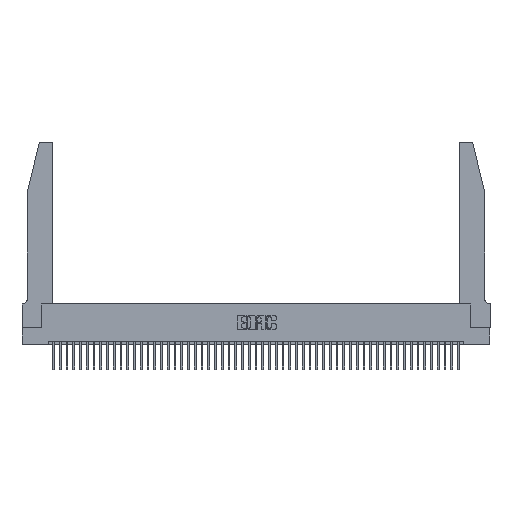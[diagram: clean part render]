
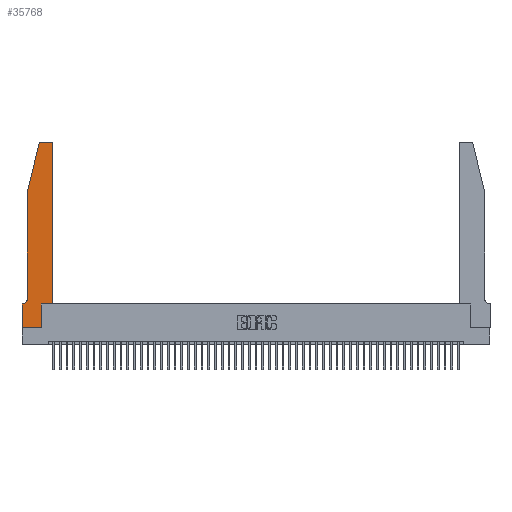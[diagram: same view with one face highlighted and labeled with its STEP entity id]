
A CAD part, top view. The second image highlights one B-rep face of the part: STEP entity #35768.
In plain terms, the highlighted planar face has unit normal (0, 0, 1).
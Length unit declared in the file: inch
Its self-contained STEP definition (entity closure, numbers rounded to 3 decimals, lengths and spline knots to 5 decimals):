
#650 = CARTESIAN_POINT ( 'NONE',  ( 0.0055, 0.42, 0.37 ) ) ;
#832 = CIRCLE ( 'NONE', #42699, 0.03 ) ;
#855 = DIRECTION ( 'NONE',  ( 1., 0., 0. ) ) ;
#888 = CARTESIAN_POINT ( 'NONE',  ( 0.284, 2.75, 0.37 ) ) ;
#952 = VERTEX_POINT ( 'NONE', #888 ) ;
#1304 = VERTEX_POINT ( 'NONE', #30046 ) ;
#1412 = VECTOR ( 'NONE', #47575, 39.37008 ) ;
#1916 = VECTOR ( 'NONE', #10757, 39.37008 ) ;
#2105 = CARTESIAN_POINT ( 'NONE',  ( 0., 0.35, 0.37 ) ) ;
#2671 = DIRECTION ( 'NONE',  ( 1., 0., 0. ) ) ;
#4132 = CARTESIAN_POINT ( 'NONE',  ( 0.0755, 2., 0.37 ) ) ;
#4643 = DIRECTION ( 'NONE',  ( -1., 0., 0. ) ) ;
#5160 = VERTEX_POINT ( 'NONE', #36260 ) ;
#5550 = ORIENTED_EDGE ( 'NONE', *, *, #30236, .T. ) ;
#7362 = CARTESIAN_POINT ( 'NONE',  ( 0.25487, 2.72718, 0.37 ) ) ;
#9404 = VERTEX_POINT ( 'NONE', #39315 ) ;
#9536 = CARTESIAN_POINT ( 'NONE',  ( 0.4205, 2.72, 0.37 ) ) ;
#9653 = AXIS2_PLACEMENT_3D ( 'NONE', #47207, #24166, #855 ) ;
#10757 = DIRECTION ( 'NONE',  ( -1., 0., 0. ) ) ;
#10974 = ORIENTED_EDGE ( 'NONE', *, *, #25733, .T. ) ;
#11867 = LINE ( 'NONE', #12893, #1412 ) ;
#12607 = FACE_OUTER_BOUND ( 'NONE', #40904, .T. ) ;
#12893 = CARTESIAN_POINT ( 'NONE',  ( 0.2865, 0.35, 0.37 ) ) ;
#13174 = LINE ( 'NONE', #13328, #23443 ) ;
#13272 = CARTESIAN_POINT ( 'NONE',  ( 0.0755, 0.42, 0.37 ) ) ;
#13328 = CARTESIAN_POINT ( 'NONE',  ( 0.4505, 0.35, 0.37 ) ) ;
#13420 = DIRECTION ( 'NONE',  ( 1., 0., 0. ) ) ;
#13622 = ORIENTED_EDGE ( 'NONE', *, *, #49044, .T. ) ;
#13881 = VERTEX_POINT ( 'NONE', #47360 ) ;
#14043 = DIRECTION ( 'NONE',  ( 0., -1., 0. ) ) ;
#14180 = AXIS2_PLACEMENT_3D ( 'NONE', #2105, #44714, #21693 ) ;
#14800 = DIRECTION ( 'NONE',  ( 0., -1., 0. ) ) ;
#15690 = LINE ( 'NONE', #17488, #34949 ) ;
#16116 = VERTEX_POINT ( 'NONE', #21688 ) ;
#16924 = VERTEX_POINT ( 'NONE', #7362 ) ;
#17362 = CIRCLE ( 'NONE', #27234, 0.07 ) ;
#17374 = EDGE_CURVE ( 'NONE', #13881, #32574, #44291, .T. ) ;
#17488 = CARTESIAN_POINT ( 'NONE',  ( 0.2605, 2.75, 0.37 ) ) ;
#17783 = VERTEX_POINT ( 'NONE', #44051 ) ;
#18094 = VERTEX_POINT ( 'NONE', #34466 ) ;
#18521 = CARTESIAN_POINT ( 'NONE',  ( 0.0755, 0.35, 0.37 ) ) ;
#18881 = CIRCLE ( 'NONE', #9653, 0.03 ) ;
#19479 = ORIENTED_EDGE ( 'NONE', *, *, #36534, .T. ) ;
#20086 = EDGE_CURVE ( 'NONE', #44939, #952, #15690, .T. ) ;
#20116 = ORIENTED_EDGE ( 'NONE', *, *, #33335, .T. ) ;
#20129 = LINE ( 'NONE', #48945, #21354 ) ;
#21072 = EDGE_CURVE ( 'NONE', #17783, #5160, #13174, .T. ) ;
#21112 = DIRECTION ( 'NONE',  ( 1., 0., 0. ) ) ;
#21149 = CARTESIAN_POINT ( 'NONE',  ( 0.4205, 2.75, 0.37 ) ) ;
#21354 = VECTOR ( 'NONE', #2671, 39.37008 ) ;
#21688 = CARTESIAN_POINT ( 'NONE',  ( 0., 0., 0.37 ) ) ;
#21693 = DIRECTION ( 'NONE',  ( 1., 0., 0. ) ) ;
#22400 = CARTESIAN_POINT ( 'NONE',  ( 0.0755, 2., 0.37 ) ) ;
#23443 = VECTOR ( 'NONE', #21112, 39.37008 ) ;
#23466 = DIRECTION ( 'NONE',  ( -0.239, -0.971, 0. ) ) ;
#24165 = VECTOR ( 'NONE', #23466, 39.37008 ) ;
#24166 = DIRECTION ( 'NONE',  ( 0., 0., 1. ) ) ;
#24174 = CARTESIAN_POINT ( 'NONE',  ( 0., 0.35, 0.37 ) ) ;
#24873 = VECTOR ( 'NONE', #25660, 39.37008 ) ;
#24995 = VERTEX_POINT ( 'NONE', #13272 ) ;
#25513 = CARTESIAN_POINT ( 'NONE',  ( 0., 0., 0.37 ) ) ;
#25660 = DIRECTION ( 'NONE',  ( 0., 1., 0. ) ) ;
#25733 = EDGE_CURVE ( 'NONE', #32574, #16116, #36470, .T. ) ;
#27234 = AXIS2_PLACEMENT_3D ( 'NONE', #650, #27822, #4643 ) ;
#27822 = DIRECTION ( 'NONE',  ( 0., 0., -1. ) ) ;
#27868 = ORIENTED_EDGE ( 'NONE', *, *, #49334, .T. ) ;
#28669 = VECTOR ( 'NONE', #14043, 39.37008 ) ;
#30046 = CARTESIAN_POINT ( 'NONE',  ( 0.2865, 0., 0.37 ) ) ;
#30100 = EDGE_CURVE ( 'NONE', #24995, #13881, #17362, .T. ) ;
#30236 = EDGE_CURVE ( 'NONE', #18094, #44939, #832, .T. ) ;
#32574 = VERTEX_POINT ( 'NONE', #24174 ) ;
#32898 = ORIENTED_EDGE ( 'NONE', *, *, #47978, .T. ) ;
#33335 = EDGE_CURVE ( 'NONE', #16116, #1304, #20129, .T. ) ;
#34466 = CARTESIAN_POINT ( 'NONE',  ( 0.4505, 2.72, 0.37 ) ) ;
#34949 = VECTOR ( 'NONE', #36811, 39.37008 ) ;
#35097 = ORIENTED_EDGE ( 'NONE', *, *, #21072, .T. ) ;
#35347 = ORIENTED_EDGE ( 'NONE', *, *, #20086, .T. ) ;
#35684 = ORIENTED_EDGE ( 'NONE', *, *, #17374, .T. ) ;
#35768 = ADVANCED_FACE ( 'NONE', ( #12607 ), #36949, .T. ) ;
#36260 = CARTESIAN_POINT ( 'NONE',  ( 0.4505, 0.35, 0.37 ) ) ;
#36469 = DIRECTION ( 'NONE',  ( 0., 0., 1. ) ) ;
#36470 = LINE ( 'NONE', #25513, #28669 ) ;
#36534 = EDGE_CURVE ( 'NONE', #1304, #17783, #11867, .T. ) ;
#36811 = DIRECTION ( 'NONE',  ( -1., 0., 0. ) ) ;
#36949 = PLANE ( 'NONE',  #14180 ) ;
#37130 = ORIENTED_EDGE ( 'NONE', *, *, #45296, .T. ) ;
#37392 = VECTOR ( 'NONE', #14800, 39.37008 ) ;
#39315 = CARTESIAN_POINT ( 'NONE',  ( 0.0755, 2., 0.37 ) ) ;
#39802 = LINE ( 'NONE', #22400, #37392 ) ;
#39938 = ORIENTED_EDGE ( 'NONE', *, *, #30100, .T. ) ;
#40904 = EDGE_LOOP ( 'NONE', ( #35347, #13622, #32898, #37130, #39938, #35684, #10974, #20116, #19479, #35097, #27868, #5550 ) ) ;
#42699 = AXIS2_PLACEMENT_3D ( 'NONE', #9536, #36469, #13420 ) ;
#44051 = CARTESIAN_POINT ( 'NONE',  ( 0.2865, 0.35, 0.37 ) ) ;
#44291 = LINE ( 'NONE', #18521, #1916 ) ;
#44714 = DIRECTION ( 'NONE',  ( 0., 0., 1. ) ) ;
#44939 = VERTEX_POINT ( 'NONE', #21149 ) ;
#45296 = EDGE_CURVE ( 'NONE', #9404, #24995, #39802, .T. ) ;
#45847 = LINE ( 'NONE', #4132, #24165 ) ;
#46555 = LINE ( 'NONE', #48516, #24873 ) ;
#47207 = CARTESIAN_POINT ( 'NONE',  ( 0.284, 2.72, 0.37 ) ) ;
#47360 = CARTESIAN_POINT ( 'NONE',  ( 0.0055, 0.35, 0.37 ) ) ;
#47575 = DIRECTION ( 'NONE',  ( 0., 1., 0. ) ) ;
#47978 = EDGE_CURVE ( 'NONE', #16924, #9404, #45847, .T. ) ;
#48516 = CARTESIAN_POINT ( 'NONE',  ( 0.4505, 0.35, 0.37 ) ) ;
#48945 = CARTESIAN_POINT ( 'NONE',  ( 0., 0., 0.37 ) ) ;
#49044 = EDGE_CURVE ( 'NONE', #952, #16924, #18881, .T. ) ;
#49334 = EDGE_CURVE ( 'NONE', #5160, #18094, #46555, .T. ) ;
